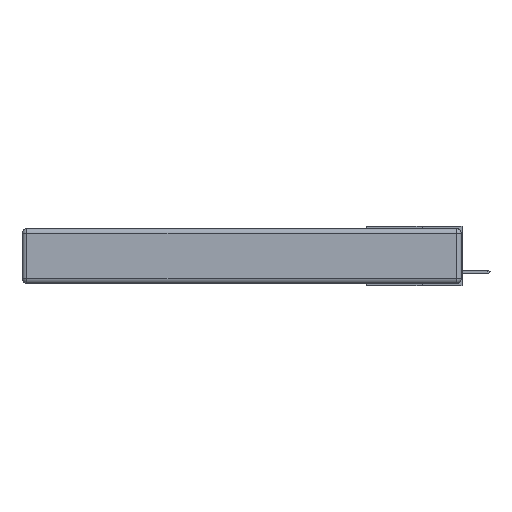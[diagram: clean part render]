
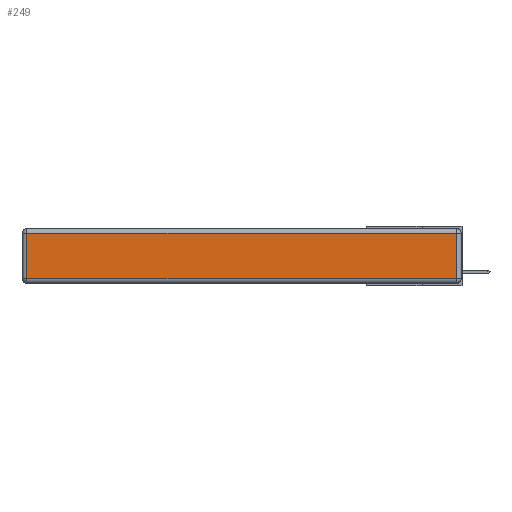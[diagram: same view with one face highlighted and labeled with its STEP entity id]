
A CAD part, left-side view. The second image highlights one B-rep face of the part: STEP entity #249.
In plain terms, the highlighted planar face has unit normal (-1, 0, 0).
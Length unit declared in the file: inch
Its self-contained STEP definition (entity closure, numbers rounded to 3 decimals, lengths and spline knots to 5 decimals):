
#7 = ORIENTED_EDGE ( 'NONE', *, *, #11201, .T. ) ;
#249 = ADVANCED_FACE ( 'NONE', ( #12270 ), #13059, .T. ) ;
#266 = ORIENTED_EDGE ( 'NONE', *, *, #7877, .T. ) ;
#844 = LINE ( 'NONE', #17164, #17113 ) ;
#1215 = EDGE_CURVE ( 'NONE', #2784, #16027, #13829, .T. ) ;
#1292 = DIRECTION ( 'NONE',  ( 0., 0., 1. ) ) ;
#1562 = LINE ( 'NONE', #9928, #18065 ) ;
#2688 = DIRECTION ( 'NONE',  ( 0., -1., 0. ) ) ;
#2784 = VERTEX_POINT ( 'NONE', #12989 ) ;
#2918 = CARTESIAN_POINT ( 'NONE',  ( 0., 0., -0.343 ) ) ;
#5718 = DIRECTION ( 'NONE',  ( 0., 0., 1. ) ) ;
#7877 = EDGE_CURVE ( 'NONE', #14209, #2784, #11583, .T. ) ;
#9256 = VERTEX_POINT ( 'NONE', #11109 ) ;
#9544 = EDGE_CURVE ( 'NONE', #9256, #14209, #1562, .T. ) ;
#9928 = CARTESIAN_POINT ( 'NONE',  ( 0., 2.75, -0.03 ) ) ;
#10293 = EDGE_LOOP ( 'NONE', ( #13482, #7, #10648, #266 ) ) ;
#10648 = ORIENTED_EDGE ( 'NONE', *, *, #9544, .T. ) ;
#11109 = CARTESIAN_POINT ( 'NONE',  ( 0., 0.03, -0.03 ) ) ;
#11201 = EDGE_CURVE ( 'NONE', #16027, #9256, #844, .T. ) ;
#11583 = LINE ( 'NONE', #15220, #18364 ) ;
#12270 = FACE_OUTER_BOUND ( 'NONE', #10293, .T. ) ;
#12719 = AXIS2_PLACEMENT_3D ( 'NONE', #2918, #18681, #5718 ) ;
#12745 = DIRECTION ( 'NONE',  ( 0., 1., 0. ) ) ;
#12989 = CARTESIAN_POINT ( 'NONE',  ( 0., 2.72, -0.313 ) ) ;
#13059 = PLANE ( 'NONE',  #12719 ) ;
#13482 = ORIENTED_EDGE ( 'NONE', *, *, #1215, .T. ) ;
#13829 = LINE ( 'NONE', #14275, #14754 ) ;
#14209 = VERTEX_POINT ( 'NONE', #17897 ) ;
#14275 = CARTESIAN_POINT ( 'NONE',  ( 0., 0., -0.313 ) ) ;
#14754 = VECTOR ( 'NONE', #2688, 39.37008 ) ;
#14964 = CARTESIAN_POINT ( 'NONE',  ( 0., 0.03, -0.313 ) ) ;
#15220 = CARTESIAN_POINT ( 'NONE',  ( 0., 2.72, -0.343 ) ) ;
#16027 = VERTEX_POINT ( 'NONE', #14964 ) ;
#16565 = DIRECTION ( 'NONE',  ( 0., 0., -1. ) ) ;
#17113 = VECTOR ( 'NONE', #1292, 39.37008 ) ;
#17164 = CARTESIAN_POINT ( 'NONE',  ( 0., 0.03, -0.343 ) ) ;
#17897 = CARTESIAN_POINT ( 'NONE',  ( 0., 2.72, -0.03 ) ) ;
#18065 = VECTOR ( 'NONE', #12745, 39.37008 ) ;
#18364 = VECTOR ( 'NONE', #16565, 39.37008 ) ;
#18681 = DIRECTION ( 'NONE',  ( -1., 0., 0. ) ) ;
